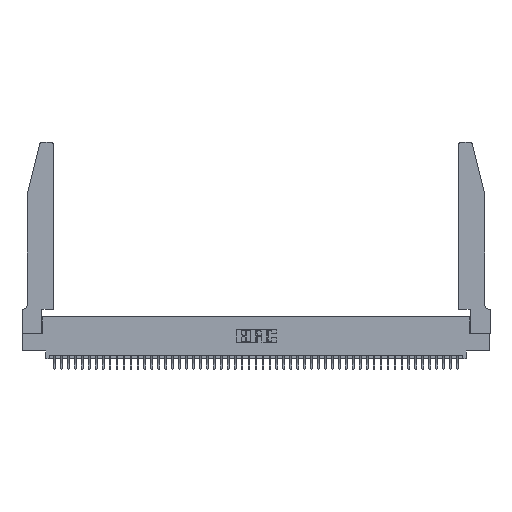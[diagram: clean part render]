
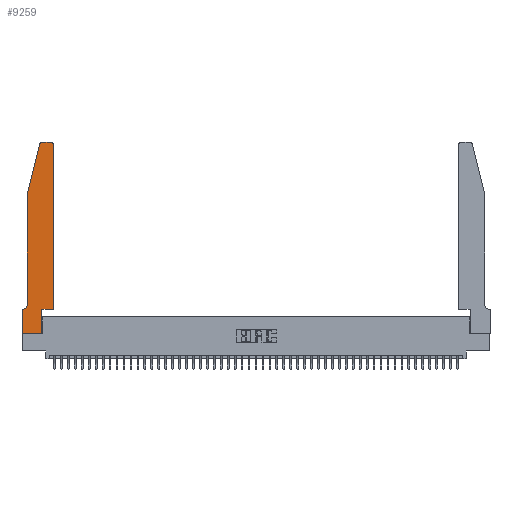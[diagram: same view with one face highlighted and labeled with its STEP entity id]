
A CAD part, top view. The second image highlights one B-rep face of the part: STEP entity #9259.
In plain terms, the highlighted planar face has unit normal (0, 0, 1).
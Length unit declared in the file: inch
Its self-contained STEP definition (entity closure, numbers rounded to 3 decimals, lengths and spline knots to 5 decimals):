
#364 = DIRECTION ( 'NONE',  ( 1., 0., 0. ) ) ;
#992 = CARTESIAN_POINT ( 'NONE',  ( 0.0755, 2., 0.37 ) ) ;
#1201 = ORIENTED_EDGE ( 'NONE', *, *, #39568, .T. ) ;
#1381 = CARTESIAN_POINT ( 'NONE',  ( 0.0755, 2., 0.37 ) ) ;
#1453 = ORIENTED_EDGE ( 'NONE', *, *, #29655, .T. ) ;
#1945 = CARTESIAN_POINT ( 'NONE',  ( 0., 0., 0.37 ) ) ;
#2700 = VERTEX_POINT ( 'NONE', #36115 ) ;
#3128 = AXIS2_PLACEMENT_3D ( 'NONE', #15932, #42453, #19773 ) ;
#3711 = VERTEX_POINT ( 'NONE', #26483 ) ;
#4007 = ORIENTED_EDGE ( 'NONE', *, *, #47663, .T. ) ;
#4047 = CARTESIAN_POINT ( 'NONE',  ( 0.0755, 0.42, 0.37 ) ) ;
#4359 = LINE ( 'NONE', #34451, #41160 ) ;
#4384 = CARTESIAN_POINT ( 'NONE',  ( 0.4205, 2.72, 0.37 ) ) ;
#4856 = ORIENTED_EDGE ( 'NONE', *, *, #23161, .T. ) ;
#5939 = VECTOR ( 'NONE', #29015, 39.37008 ) ;
#7150 = LINE ( 'NONE', #21556, #5939 ) ;
#7448 = AXIS2_PLACEMENT_3D ( 'NONE', #26846, #23197, #364 ) ;
#8019 = CARTESIAN_POINT ( 'NONE',  ( 0.0755, 0.35, 0.37 ) ) ;
#8023 = EDGE_CURVE ( 'NONE', #37814, #9314, #16914, .T. ) ;
#8039 = CARTESIAN_POINT ( 'NONE',  ( 0.4505, 0.35, 0.37 ) ) ;
#8197 = DIRECTION ( 'NONE',  ( 1., 0., 0. ) ) ;
#8450 = DIRECTION ( 'NONE',  ( 1., 0., 0. ) ) ;
#9259 = ADVANCED_FACE ( 'NONE', ( #13190 ), #19339, .T. ) ;
#9264 = EDGE_CURVE ( 'NONE', #2700, #47236, #31065, .T. ) ;
#9314 = VERTEX_POINT ( 'NONE', #19675 ) ;
#10397 = ORIENTED_EDGE ( 'NONE', *, *, #32966, .T. ) ;
#12087 = VERTEX_POINT ( 'NONE', #36056 ) ;
#12537 = ORIENTED_EDGE ( 'NONE', *, *, #45497, .T. ) ;
#13190 = FACE_OUTER_BOUND ( 'NONE', #30049, .T. ) ;
#13256 = DIRECTION ( 'NONE',  ( 0., -1., 0. ) ) ;
#13616 = LINE ( 'NONE', #1945, #42691 ) ;
#13618 = CARTESIAN_POINT ( 'NONE',  ( 0.0755, 2., 0.37 ) ) ;
#14405 = AXIS2_PLACEMENT_3D ( 'NONE', #42744, #20078, #46552 ) ;
#15275 = CIRCLE ( 'NONE', #18180, 0.03 ) ;
#15530 = DIRECTION ( 'NONE',  ( 0., 1., 0. ) ) ;
#15932 = CARTESIAN_POINT ( 'NONE',  ( 0.0055, 0.42, 0.37 ) ) ;
#15934 = CARTESIAN_POINT ( 'NONE',  ( 0., 0., 0.37 ) ) ;
#16039 = VECTOR ( 'NONE', #16290, 39.37008 ) ;
#16290 = DIRECTION ( 'NONE',  ( -0.239, -0.971, 0. ) ) ;
#16910 = EDGE_CURVE ( 'NONE', #20191, #46351, #46279, .T. ) ;
#16914 = LINE ( 'NONE', #15934, #25883 ) ;
#17380 = VERTEX_POINT ( 'NONE', #22777 ) ;
#18180 = AXIS2_PLACEMENT_3D ( 'NONE', #4384, #31011, #8197 ) ;
#19014 = ORIENTED_EDGE ( 'NONE', *, *, #9264, .T. ) ;
#19063 = CARTESIAN_POINT ( 'NONE',  ( 0.2865, 0.35, 0.37 ) ) ;
#19339 = PLANE ( 'NONE',  #7448 ) ;
#19675 = CARTESIAN_POINT ( 'NONE',  ( 0.2865, 0., 0.37 ) ) ;
#19773 = DIRECTION ( 'NONE',  ( -1., 0., 0. ) ) ;
#20078 = DIRECTION ( 'NONE',  ( 0., 0., 1. ) ) ;
#20191 = VERTEX_POINT ( 'NONE', #38982 ) ;
#20744 = EDGE_CURVE ( 'NONE', #9314, #44079, #4359, .T. ) ;
#20784 = EDGE_CURVE ( 'NONE', #44079, #12087, #31146, .T. ) ;
#20964 = CARTESIAN_POINT ( 'NONE',  ( 0.4505, 0.35, 0.37 ) ) ;
#21086 = VECTOR ( 'NONE', #32560, 39.37008 ) ;
#21196 = VECTOR ( 'NONE', #39828, 39.37008 ) ;
#21538 = ORIENTED_EDGE ( 'NONE', *, *, #16910, .T. ) ;
#21556 = CARTESIAN_POINT ( 'NONE',  ( 0.2605, 2.75, 0.37 ) ) ;
#22276 = LINE ( 'NONE', #13618, #21086 ) ;
#22777 = CARTESIAN_POINT ( 'NONE',  ( 0.4205, 2.75, 0.37 ) ) ;
#23130 = VERTEX_POINT ( 'NONE', #4047 ) ;
#23161 = EDGE_CURVE ( 'NONE', #23762, #17380, #15275, .T. ) ;
#23197 = DIRECTION ( 'NONE',  ( 0., 0., 1. ) ) ;
#23446 = CIRCLE ( 'NONE', #3128, 0.07 ) ;
#23762 = VERTEX_POINT ( 'NONE', #34548 ) ;
#24530 = EDGE_CURVE ( 'NONE', #3711, #20191, #37699, .T. ) ;
#25883 = VECTOR ( 'NONE', #8450, 39.37008 ) ;
#26138 = CARTESIAN_POINT ( 'NONE',  ( 0., 0.35, 0.37 ) ) ;
#26483 = CARTESIAN_POINT ( 'NONE',  ( 0.284, 2.75, 0.37 ) ) ;
#26846 = CARTESIAN_POINT ( 'NONE',  ( 0., 0.35, 0.37 ) ) ;
#27449 = CARTESIAN_POINT ( 'NONE',  ( 0., 0., 0.37 ) ) ;
#29015 = DIRECTION ( 'NONE',  ( -1., 0., 0. ) ) ;
#29655 = EDGE_CURVE ( 'NONE', #12087, #23762, #41317, .T. ) ;
#30049 = EDGE_LOOP ( 'NONE', ( #10397, #41327, #21538, #1201, #12537, #19014, #4007, #31953, #35983, #47039, #1453, #4856 ) ) ;
#31011 = DIRECTION ( 'NONE',  ( 0., 0., 1. ) ) ;
#31065 = LINE ( 'NONE', #8019, #42266 ) ;
#31146 = LINE ( 'NONE', #8039, #39980 ) ;
#31953 = ORIENTED_EDGE ( 'NONE', *, *, #8023, .T. ) ;
#32560 = DIRECTION ( 'NONE',  ( 0., -1., 0. ) ) ;
#32966 = EDGE_CURVE ( 'NONE', #17380, #3711, #7150, .T. ) ;
#34451 = CARTESIAN_POINT ( 'NONE',  ( 0.2865, 0.35, 0.37 ) ) ;
#34548 = CARTESIAN_POINT ( 'NONE',  ( 0.4505, 2.72, 0.37 ) ) ;
#34589 = DIRECTION ( 'NONE',  ( -1., 0., 0. ) ) ;
#35983 = ORIENTED_EDGE ( 'NONE', *, *, #20744, .T. ) ;
#36056 = CARTESIAN_POINT ( 'NONE',  ( 0.4505, 0.35, 0.37 ) ) ;
#36115 = CARTESIAN_POINT ( 'NONE',  ( 0.0055, 0.35, 0.37 ) ) ;
#37699 = CIRCLE ( 'NONE', #14405, 0.03 ) ;
#37814 = VERTEX_POINT ( 'NONE', #27449 ) ;
#38422 = DIRECTION ( 'NONE',  ( 1., 0., 0. ) ) ;
#38982 = CARTESIAN_POINT ( 'NONE',  ( 0.25487, 2.72718, 0.37 ) ) ;
#39568 = EDGE_CURVE ( 'NONE', #46351, #23130, #22276, .T. ) ;
#39828 = DIRECTION ( 'NONE',  ( 0., 1., 0. ) ) ;
#39980 = VECTOR ( 'NONE', #38422, 39.37008 ) ;
#41160 = VECTOR ( 'NONE', #15530, 39.37008 ) ;
#41317 = LINE ( 'NONE', #20964, #21196 ) ;
#41327 = ORIENTED_EDGE ( 'NONE', *, *, #24530, .T. ) ;
#42266 = VECTOR ( 'NONE', #34589, 39.37008 ) ;
#42453 = DIRECTION ( 'NONE',  ( 0., 0., -1. ) ) ;
#42691 = VECTOR ( 'NONE', #13256, 39.37008 ) ;
#42744 = CARTESIAN_POINT ( 'NONE',  ( 0.284, 2.72, 0.37 ) ) ;
#44079 = VERTEX_POINT ( 'NONE', #19063 ) ;
#45497 = EDGE_CURVE ( 'NONE', #23130, #2700, #23446, .T. ) ;
#46279 = LINE ( 'NONE', #992, #16039 ) ;
#46351 = VERTEX_POINT ( 'NONE', #1381 ) ;
#46552 = DIRECTION ( 'NONE',  ( 1., 0., 0. ) ) ;
#47039 = ORIENTED_EDGE ( 'NONE', *, *, #20784, .T. ) ;
#47236 = VERTEX_POINT ( 'NONE', #26138 ) ;
#47663 = EDGE_CURVE ( 'NONE', #47236, #37814, #13616, .T. ) ;
